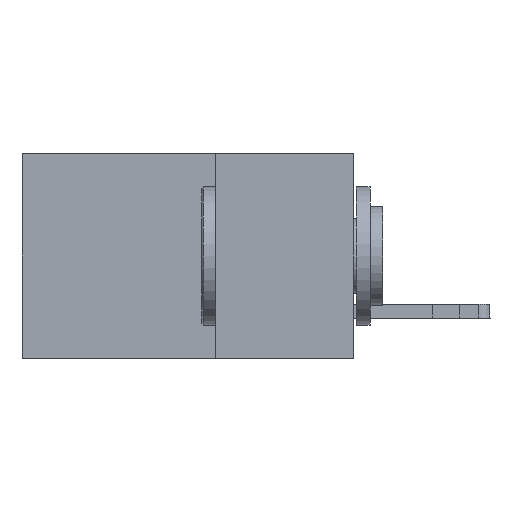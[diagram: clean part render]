
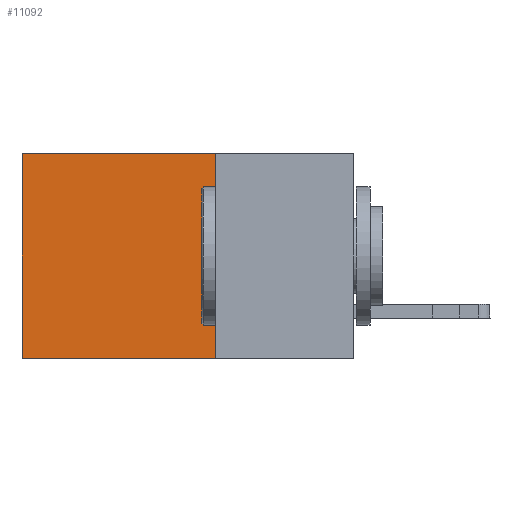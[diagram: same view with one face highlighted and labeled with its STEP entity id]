
A CAD part, left-side view. The second image highlights one B-rep face of the part: STEP entity #11092.
In plain terms, the highlighted planar face has unit normal (-1, 0, 0).
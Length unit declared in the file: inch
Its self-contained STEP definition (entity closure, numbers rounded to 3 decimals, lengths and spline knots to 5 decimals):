
#243 = CARTESIAN_POINT ( 'NONE',  ( 0.2875, 0.25, 0. ) ) ;
#549 = VERTEX_POINT ( 'NONE', #841 ) ;
#693 = VERTEX_POINT ( 'NONE', #1755 ) ;
#841 = CARTESIAN_POINT ( 'NONE',  ( 0.2875, 0.6, 0. ) ) ;
#1726 = EDGE_LOOP ( 'NONE', ( #4938, #11422, #7210, #17315 ) ) ;
#1755 = CARTESIAN_POINT ( 'NONE',  ( 0.2875, 0.6, -0.37 ) ) ;
#3214 = LINE ( 'NONE', #13284, #10450 ) ;
#3224 = DIRECTION ( 'NONE',  ( 0., 0., -1. ) ) ;
#3659 = CARTESIAN_POINT ( 'NONE',  ( 0.2875, 0.25, 0. ) ) ;
#4136 = EDGE_CURVE ( 'NONE', #17016, #8394, #4944, .T. ) ;
#4492 = EDGE_CURVE ( 'NONE', #17016, #549, #10117, .T. ) ;
#4617 = FACE_OUTER_BOUND ( 'NONE', #1726, .T. ) ;
#4938 = ORIENTED_EDGE ( 'NONE', *, *, #12465, .T. ) ;
#4944 = LINE ( 'NONE', #3659, #12194 ) ;
#5204 = EDGE_CURVE ( 'NONE', #8394, #693, #17424, .T. ) ;
#5523 = AXIS2_PLACEMENT_3D ( 'NONE', #243, #11886, #3224 ) ;
#6071 = DIRECTION ( 'NONE',  ( 0., 0., -1. ) ) ;
#6708 = CARTESIAN_POINT ( 'NONE',  ( 0.2875, 0.25, -0.37 ) ) ;
#7210 = ORIENTED_EDGE ( 'NONE', *, *, #4136, .F. ) ;
#8394 = VERTEX_POINT ( 'NONE', #6708 ) ;
#10117 = LINE ( 'NONE', #13372, #17236 ) ;
#10450 = VECTOR ( 'NONE', #6071, 39.37008 ) ;
#10864 = DIRECTION ( 'NONE',  ( 0., 0., -1. ) ) ;
#11092 = ADVANCED_FACE ( 'NONE', ( #4617 ), #16100, .F. ) ;
#11422 = ORIENTED_EDGE ( 'NONE', *, *, #5204, .F. ) ;
#11886 = DIRECTION ( 'NONE',  ( 1., 0., 0. ) ) ;
#11967 = DIRECTION ( 'NONE',  ( 0., 1., 0. ) ) ;
#12194 = VECTOR ( 'NONE', #10864, 39.37008 ) ;
#12465 = EDGE_CURVE ( 'NONE', #549, #693, #3214, .T. ) ;
#13253 = VECTOR ( 'NONE', #11967, 39.37008 ) ;
#13284 = CARTESIAN_POINT ( 'NONE',  ( 0.2875, 0.6, 0. ) ) ;
#13308 = DIRECTION ( 'NONE',  ( 0., 1., 0. ) ) ;
#13372 = CARTESIAN_POINT ( 'NONE',  ( 0.2875, 0.25, 0. ) ) ;
#14809 = CARTESIAN_POINT ( 'NONE',  ( 0.2875, 0.25, -0.37 ) ) ;
#14979 = CARTESIAN_POINT ( 'NONE',  ( 0.2875, 0.25, 0. ) ) ;
#16100 = PLANE ( 'NONE',  #5523 ) ;
#17016 = VERTEX_POINT ( 'NONE', #14979 ) ;
#17236 = VECTOR ( 'NONE', #13308, 39.37008 ) ;
#17315 = ORIENTED_EDGE ( 'NONE', *, *, #4492, .T. ) ;
#17424 = LINE ( 'NONE', #14809, #13253 ) ;
